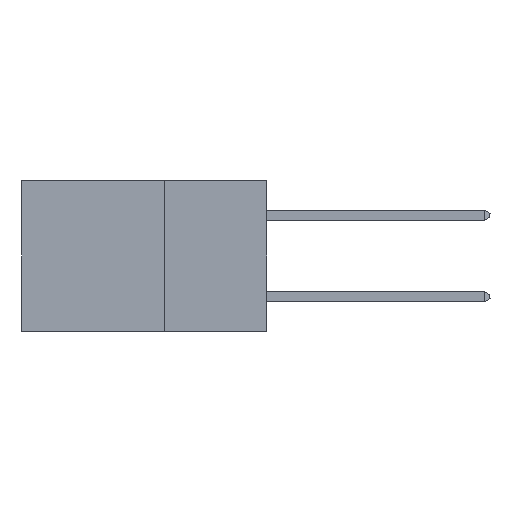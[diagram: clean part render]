
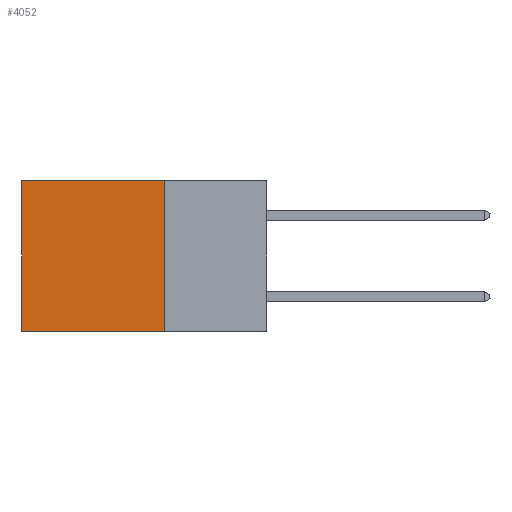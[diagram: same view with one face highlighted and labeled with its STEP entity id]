
A CAD part, left-side view. The second image highlights one B-rep face of the part: STEP entity #4052.
In plain terms, the highlighted planar face has unit normal (-1, 0, 0).
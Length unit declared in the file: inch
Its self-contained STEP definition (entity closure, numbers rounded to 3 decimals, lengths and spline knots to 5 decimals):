
#215 = EDGE_CURVE ( 'NONE', #26248, #28606, #35330, .T. ) ;
#1246 = CARTESIAN_POINT ( 'NONE',  ( 0.2875, 0.6, 0. ) ) ;
#1951 = EDGE_CURVE ( 'NONE', #26248, #37086, #10382, .T. ) ;
#2194 = VERTEX_POINT ( 'NONE', #32202 ) ;
#2726 = VECTOR ( 'NONE', #21205, 39.37008 ) ;
#3179 = LINE ( 'NONE', #15160, #2726 ) ;
#3263 = ORIENTED_EDGE ( 'NONE', *, *, #35372, .T. ) ;
#4052 = ADVANCED_FACE ( 'NONE', ( #15398 ), #5454, .F. ) ;
#5454 = PLANE ( 'NONE',  #6958 ) ;
#6958 = AXIS2_PLACEMENT_3D ( 'NONE', #35180, #20300, #24414 ) ;
#8252 = DIRECTION ( 'NONE',  ( 0., 0., -1. ) ) ;
#10382 = LINE ( 'NONE', #25426, #27683 ) ;
#14613 = CARTESIAN_POINT ( 'NONE',  ( 0.2875, 0.25, -0.37 ) ) ;
#15160 = CARTESIAN_POINT ( 'NONE',  ( 0.2875, 0.6, 0. ) ) ;
#15398 = FACE_OUTER_BOUND ( 'NONE', #35380, .T. ) ;
#15929 = CARTESIAN_POINT ( 'NONE',  ( 0.2875, 0.25, -0.37 ) ) ;
#19113 = EDGE_CURVE ( 'NONE', #37086, #2194, #31922, .T. ) ;
#19340 = ORIENTED_EDGE ( 'NONE', *, *, #1951, .F. ) ;
#20300 = DIRECTION ( 'NONE',  ( 1., 0., 0. ) ) ;
#20985 = CARTESIAN_POINT ( 'NONE',  ( 0.2875, 0.25, 0. ) ) ;
#21205 = DIRECTION ( 'NONE',  ( 0., 0., -1. ) ) ;
#22809 = ORIENTED_EDGE ( 'NONE', *, *, #215, .T. ) ;
#24414 = DIRECTION ( 'NONE',  ( 0., 0., -1. ) ) ;
#25344 = DIRECTION ( 'NONE',  ( 0., 1., 0. ) ) ;
#25426 = CARTESIAN_POINT ( 'NONE',  ( 0.2875, 0.25, 0. ) ) ;
#25575 = CARTESIAN_POINT ( 'NONE',  ( 0.2875, 0.25, 0. ) ) ;
#26248 = VERTEX_POINT ( 'NONE', #20985 ) ;
#27683 = VECTOR ( 'NONE', #8252, 39.37008 ) ;
#28317 = VECTOR ( 'NONE', #38031, 39.37008 ) ;
#28606 = VERTEX_POINT ( 'NONE', #1246 ) ;
#31922 = LINE ( 'NONE', #15929, #36637 ) ;
#32202 = CARTESIAN_POINT ( 'NONE',  ( 0.2875, 0.6, -0.37 ) ) ;
#35180 = CARTESIAN_POINT ( 'NONE',  ( 0.2875, 0.25, 0. ) ) ;
#35330 = LINE ( 'NONE', #25575, #28317 ) ;
#35372 = EDGE_CURVE ( 'NONE', #28606, #2194, #3179, .T. ) ;
#35380 = EDGE_LOOP ( 'NONE', ( #3263, #36494, #19340, #22809 ) ) ;
#36494 = ORIENTED_EDGE ( 'NONE', *, *, #19113, .F. ) ;
#36637 = VECTOR ( 'NONE', #25344, 39.37008 ) ;
#37086 = VERTEX_POINT ( 'NONE', #14613 ) ;
#38031 = DIRECTION ( 'NONE',  ( 0., 1., 0. ) ) ;
